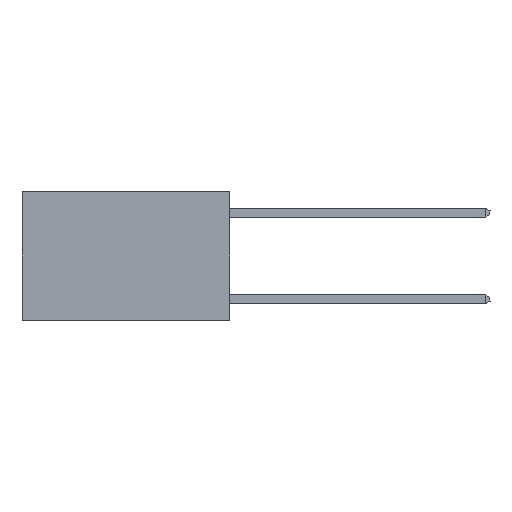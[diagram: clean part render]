
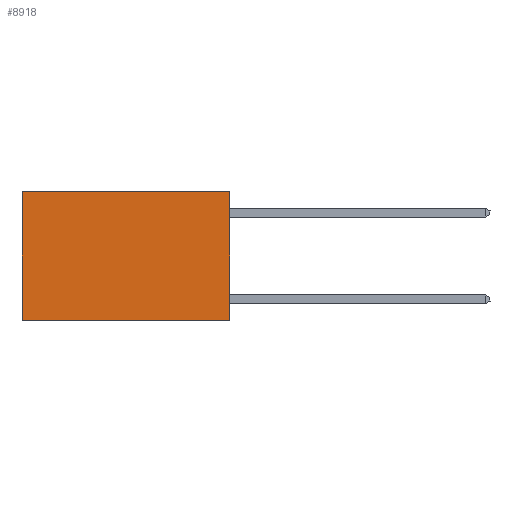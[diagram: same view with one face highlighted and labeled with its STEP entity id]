
A CAD part, left-side view. The second image highlights one B-rep face of the part: STEP entity #8918.
In plain terms, the highlighted planar face has unit normal (-1, 0, 0).
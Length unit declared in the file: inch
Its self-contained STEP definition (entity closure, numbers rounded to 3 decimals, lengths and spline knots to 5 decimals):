
#871 = ORIENTED_EDGE ( 'NONE', *, *, #7159, .F. ) ;
#1617 = DIRECTION ( 'NONE',  ( 0., 1., 0. ) ) ;
#1959 = EDGE_CURVE ( 'NONE', #8474, #8650, #16949, .T. ) ;
#2014 = CARTESIAN_POINT ( 'NONE',  ( 0.2625, 0.6, -0.37 ) ) ;
#2520 = CARTESIAN_POINT ( 'NONE',  ( 0.2625, 0., 0. ) ) ;
#3408 = VECTOR ( 'NONE', #1617, 39.37008 ) ;
#4505 = CARTESIAN_POINT ( 'NONE',  ( 0.2625, 0., 0. ) ) ;
#4781 = DIRECTION ( 'NONE',  ( 0., 0., -1. ) ) ;
#5099 = CARTESIAN_POINT ( 'NONE',  ( 0.2625, 0.6, 0. ) ) ;
#5527 = CARTESIAN_POINT ( 'NONE',  ( 0.2625, 0.6, 0. ) ) ;
#6312 = LINE ( 'NONE', #15528, #3408 ) ;
#6334 = LINE ( 'NONE', #2520, #10970 ) ;
#6767 = DIRECTION ( 'NONE',  ( 0., 1., 0. ) ) ;
#7159 = EDGE_CURVE ( 'NONE', #8650, #12886, #6312, .T. ) ;
#7843 = ORIENTED_EDGE ( 'NONE', *, *, #1959, .F. ) ;
#8474 = VERTEX_POINT ( 'NONE', #16108 ) ;
#8650 = VERTEX_POINT ( 'NONE', #10728 ) ;
#8918 = ADVANCED_FACE ( 'NONE', ( #18015 ), #11812, .F. ) ;
#9642 = EDGE_LOOP ( 'NONE', ( #11811, #871, #7843, #13050 ) ) ;
#10728 = CARTESIAN_POINT ( 'NONE',  ( 0.2625, 0., -0.37 ) ) ;
#10970 = VECTOR ( 'NONE', #6767, 39.37008 ) ;
#11482 = DIRECTION ( 'NONE',  ( 0., 0., -1. ) ) ;
#11811 = ORIENTED_EDGE ( 'NONE', *, *, #13708, .T. ) ;
#11812 = PLANE ( 'NONE',  #14534 ) ;
#12446 = EDGE_CURVE ( 'NONE', #8474, #14060, #6334, .T. ) ;
#12517 = LINE ( 'NONE', #5099, #17388 ) ;
#12886 = VERTEX_POINT ( 'NONE', #2014 ) ;
#13050 = ORIENTED_EDGE ( 'NONE', *, *, #12446, .T. ) ;
#13708 = EDGE_CURVE ( 'NONE', #14060, #12886, #12517, .T. ) ;
#14060 = VERTEX_POINT ( 'NONE', #5527 ) ;
#14079 = VECTOR ( 'NONE', #11482, 39.37008 ) ;
#14516 = CARTESIAN_POINT ( 'NONE',  ( 0.2625, 0., 0. ) ) ;
#14534 = AXIS2_PLACEMENT_3D ( 'NONE', #14516, #14572, #4781 ) ;
#14572 = DIRECTION ( 'NONE',  ( 1., 0., 0. ) ) ;
#15528 = CARTESIAN_POINT ( 'NONE',  ( 0.2625, 0., -0.37 ) ) ;
#16108 = CARTESIAN_POINT ( 'NONE',  ( 0.2625, 0., 0. ) ) ;
#16949 = LINE ( 'NONE', #4505, #14079 ) ;
#17388 = VECTOR ( 'NONE', #17918, 39.37008 ) ;
#17918 = DIRECTION ( 'NONE',  ( 0., 0., -1. ) ) ;
#18015 = FACE_OUTER_BOUND ( 'NONE', #9642, .T. ) ;
